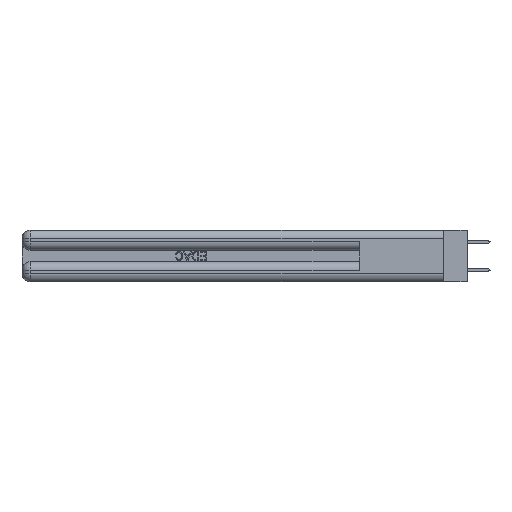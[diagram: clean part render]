
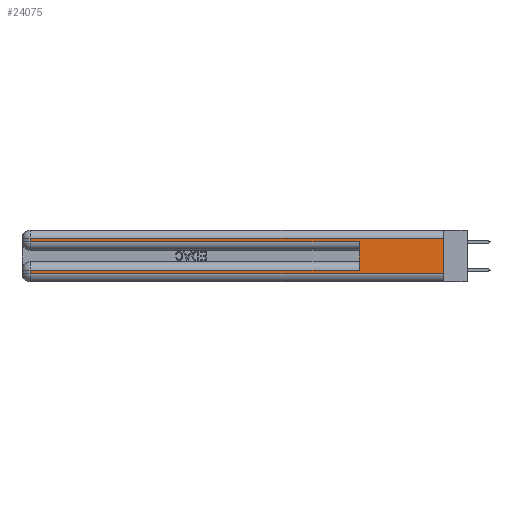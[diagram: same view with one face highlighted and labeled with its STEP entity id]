
A CAD part, left-side view. The second image highlights one B-rep face of the part: STEP entity #24075.
In plain terms, the highlighted planar face has unit normal (-1, 0, 0).
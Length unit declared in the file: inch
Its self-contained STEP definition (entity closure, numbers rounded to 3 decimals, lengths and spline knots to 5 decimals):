
#1249 = DIRECTION ( 'NONE',  ( 0., 0., -1. ) ) ;
#1422 = EDGE_CURVE ( 'NONE', #4118, #7346, #22750, .T. ) ;
#2330 = EDGE_CURVE ( 'NONE', #7348, #6141, #39832, .T. ) ;
#4068 = ORIENTED_EDGE ( 'NONE', *, *, #34071, .F. ) ;
#4118 = VERTEX_POINT ( 'NONE', #7821 ) ;
#5358 = VERTEX_POINT ( 'NONE', #38046 ) ;
#5602 = ORIENTED_EDGE ( 'NONE', *, *, #26731, .T. ) ;
#6141 = VERTEX_POINT ( 'NONE', #31432 ) ;
#6375 = CARTESIAN_POINT ( 'NONE',  ( 0., 0., 0.085 ) ) ;
#6661 = DIRECTION ( 'NONE',  ( 0., 1., 0. ) ) ;
#7010 = VERTEX_POINT ( 'NONE', #22128 ) ;
#7296 = CARTESIAN_POINT ( 'NONE',  ( 0., 0., 0.285 ) ) ;
#7346 = VERTEX_POINT ( 'NONE', #36303 ) ;
#7348 = VERTEX_POINT ( 'NONE', #32839 ) ;
#7821 = CARTESIAN_POINT ( 'NONE',  ( 0., 0.6, 0.085 ) ) ;
#8356 = LINE ( 'NONE', #32702, #28082 ) ;
#9148 = EDGE_LOOP ( 'NONE', ( #4068, #19992, #23038, #36407, #20126, #42732, #5602, #10421 ) ) ;
#9287 = VECTOR ( 'NONE', #39353, 39.37008 ) ;
#10421 = ORIENTED_EDGE ( 'NONE', *, *, #30011, .T. ) ;
#11472 = PLANE ( 'NONE',  #24019 ) ;
#11950 = DIRECTION ( 'NONE',  ( 0., -1., 0. ) ) ;
#12208 = CARTESIAN_POINT ( 'NONE',  ( 0., 2.94, 0.085 ) ) ;
#12829 = DIRECTION ( 'NONE',  ( 0., 0., -1. ) ) ;
#12841 = VECTOR ( 'NONE', #22559, 39.37008 ) ;
#13881 = VECTOR ( 'NONE', #28757, 39.37008 ) ;
#15444 = LINE ( 'NONE', #6375, #32085 ) ;
#18091 = DIRECTION ( 'NONE',  ( 1., 0., 0. ) ) ;
#18191 = CARTESIAN_POINT ( 'NONE',  ( 0., 2.94, 0.37 ) ) ;
#19479 = VECTOR ( 'NONE', #1249, 39.37008 ) ;
#19992 = ORIENTED_EDGE ( 'NONE', *, *, #2330, .T. ) ;
#20126 = ORIENTED_EDGE ( 'NONE', *, *, #1422, .F. ) ;
#21082 = VERTEX_POINT ( 'NONE', #12208 ) ;
#21270 = VECTOR ( 'NONE', #27467, 39.37008 ) ;
#22128 = CARTESIAN_POINT ( 'NONE',  ( 0., 2.94, 0.06 ) ) ;
#22559 = DIRECTION ( 'NONE',  ( 0., 1., 0. ) ) ;
#22750 = LINE ( 'NONE', #38313, #13881 ) ;
#23038 = ORIENTED_EDGE ( 'NONE', *, *, #29168, .T. ) ;
#23854 = LINE ( 'NONE', #7296, #21270 ) ;
#24019 = AXIS2_PLACEMENT_3D ( 'NONE', #31043, #18091, #27552 ) ;
#24075 = ADVANCED_FACE ( 'NONE', ( #37398 ), #11472, .F. ) ;
#25631 = LINE ( 'NONE', #41930, #29283 ) ;
#25883 = CARTESIAN_POINT ( 'NONE',  ( 0., 2.94, 0.37 ) ) ;
#26390 = EDGE_CURVE ( 'NONE', #5358, #7346, #23854, .T. ) ;
#26468 = CARTESIAN_POINT ( 'NONE',  ( 0., 0., 0.31 ) ) ;
#26731 = EDGE_CURVE ( 'NONE', #21082, #7010, #28536, .T. ) ;
#27467 = DIRECTION ( 'NONE',  ( 0., -1., 0. ) ) ;
#27552 = DIRECTION ( 'NONE',  ( 0., 0., -1. ) ) ;
#28082 = VECTOR ( 'NONE', #12829, 39.37008 ) ;
#28224 = CARTESIAN_POINT ( 'NONE',  ( 0., 0., 0.06 ) ) ;
#28536 = LINE ( 'NONE', #25883, #9287 ) ;
#28757 = DIRECTION ( 'NONE',  ( 0., 0., 1. ) ) ;
#29168 = EDGE_CURVE ( 'NONE', #6141, #5358, #39717, .T. ) ;
#29283 = VECTOR ( 'NONE', #11950, 39.37008 ) ;
#30011 = EDGE_CURVE ( 'NONE', #7010, #34876, #25631, .T. ) ;
#31043 = CARTESIAN_POINT ( 'NONE',  ( 0., 0., 0.37 ) ) ;
#31432 = CARTESIAN_POINT ( 'NONE',  ( 0., 2.94, 0.31 ) ) ;
#32085 = VECTOR ( 'NONE', #6661, 39.37008 ) ;
#32702 = CARTESIAN_POINT ( 'NONE',  ( 0., 0., 0.37 ) ) ;
#32839 = CARTESIAN_POINT ( 'NONE',  ( 0., 0., 0.31 ) ) ;
#34071 = EDGE_CURVE ( 'NONE', #7348, #34876, #8356, .T. ) ;
#34876 = VERTEX_POINT ( 'NONE', #28224 ) ;
#35823 = EDGE_CURVE ( 'NONE', #4118, #21082, #15444, .T. ) ;
#36303 = CARTESIAN_POINT ( 'NONE',  ( 0., 0.6, 0.285 ) ) ;
#36407 = ORIENTED_EDGE ( 'NONE', *, *, #26390, .T. ) ;
#37398 = FACE_OUTER_BOUND ( 'NONE', #9148, .T. ) ;
#38046 = CARTESIAN_POINT ( 'NONE',  ( 0., 2.94, 0.285 ) ) ;
#38313 = CARTESIAN_POINT ( 'NONE',  ( 0., 0.6, 0.145 ) ) ;
#39353 = DIRECTION ( 'NONE',  ( 0., 0., -1. ) ) ;
#39717 = LINE ( 'NONE', #18191, #19479 ) ;
#39832 = LINE ( 'NONE', #26468, #12841 ) ;
#41930 = CARTESIAN_POINT ( 'NONE',  ( 0., 0., 0.06 ) ) ;
#42732 = ORIENTED_EDGE ( 'NONE', *, *, #35823, .T. ) ;
